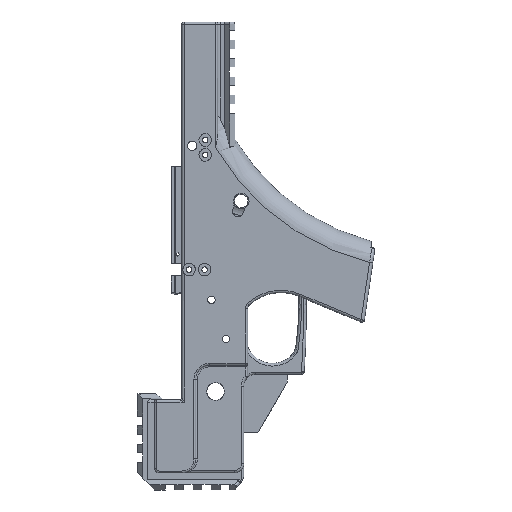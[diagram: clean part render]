
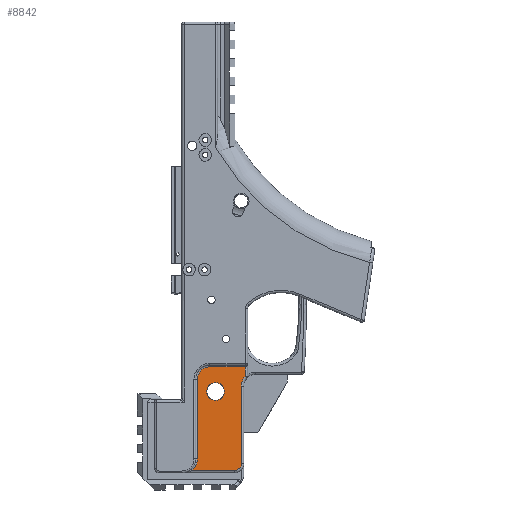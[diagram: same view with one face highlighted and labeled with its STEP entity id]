
A CAD part, left-side view. The second image highlights one B-rep face of the part: STEP entity #8842.
In plain terms, the highlighted planar face has unit normal (-1, 0, 0).
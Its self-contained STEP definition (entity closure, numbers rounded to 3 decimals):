
#143=FACE_BOUND('',#1619,.T.);
#611=CIRCLE('',#9327,7.62);
#613=CIRCLE('',#9331,3.81);
#632=CIRCLE('',#9359,6.752);
#637=CIRCLE('',#9367,8.488);
#704=CIRCLE('',#9526,4.826);
#1105=FACE_OUTER_BOUND('',#1618,.T.);
#1618=EDGE_LOOP('',(#6726,#6727,#6728,#6729,#6730,#6731,#6732,#6733,#6734));
#1619=EDGE_LOOP('',(#6735));
#2211=LINE('',#13867,#2984);
#2214=LINE('',#13884,#2987);
#2218=LINE('',#13924,#2991);
#2220=LINE('',#13937,#2993);
#2417=LINE('',#15144,#3190);
#2984=VECTOR('',#10611,10.);
#2987=VECTOR('',#10626,10.);
#2991=VECTOR('',#10670,10.);
#2993=VECTOR('',#10686,10.);
#3190=VECTOR('',#11211,10.);
#3818=VERTEX_POINT('',#13858);
#3820=VERTEX_POINT('',#13862);
#3821=VERTEX_POINT('',#13866);
#3823=VERTEX_POINT('',#13872);
#3825=VERTEX_POINT('',#13878);
#3840=VERTEX_POINT('',#13921);
#3841=VERTEX_POINT('',#13923);
#3843=VERTEX_POINT('',#13929);
#3845=VERTEX_POINT('',#13935);
#4061=VERTEX_POINT('',#15145);
#4747=EDGE_CURVE('',#3820,#3818,#611,.T.);
#4748=EDGE_CURVE('',#3818,#3821,#2211,.T.);
#4751=EDGE_CURVE('',#3821,#3823,#613,.T.);
#4756=EDGE_CURVE('',#3823,#3825,#2214,.T.);
#4773=EDGE_CURVE('',#3840,#3841,#2218,.T.);
#4777=EDGE_CURVE('',#3843,#3840,#632,.T.);
#4780=EDGE_CURVE('',#3845,#3843,#2220,.T.);
#4786=EDGE_CURVE('',#3825,#3845,#637,.T.);
#5090=EDGE_CURVE('',#3841,#3820,#2417,.T.);
#5091=EDGE_CURVE('',#4061,#4061,#704,.T.);
#6726=ORIENTED_EDGE('',*,*,#4747,.F.);
#6727=ORIENTED_EDGE('',*,*,#5090,.F.);
#6728=ORIENTED_EDGE('',*,*,#4773,.F.);
#6729=ORIENTED_EDGE('',*,*,#4777,.F.);
#6730=ORIENTED_EDGE('',*,*,#4780,.F.);
#6731=ORIENTED_EDGE('',*,*,#4786,.F.);
#6732=ORIENTED_EDGE('',*,*,#4756,.F.);
#6733=ORIENTED_EDGE('',*,*,#4751,.F.);
#6734=ORIENTED_EDGE('',*,*,#4748,.F.);
#6735=ORIENTED_EDGE('',*,*,#5091,.T.);
#8541=PLANE('',#9525);
#8842=ADVANCED_FACE('',(#1105,#143),#8541,.F.);
#9327=AXIS2_PLACEMENT_3D('',#13864,#10607,#10608);
#9331=AXIS2_PLACEMENT_3D('',#13873,#10617,#10618);
#9359=AXIS2_PLACEMENT_3D('',#13931,#10679,#10680);
#9367=AXIS2_PLACEMENT_3D('',#13970,#10698,#10699);
#9525=AXIS2_PLACEMENT_3D('',#15143,#11209,#11210);
#9526=AXIS2_PLACEMENT_3D('',#15146,#11212,#11213);
#10607=DIRECTION('center_axis',(-1.,0.,0.));
#10608=DIRECTION('ref_axis',(0.,0.928,0.373));
#10611=DIRECTION('',(0.,0.,-1.));
#10617=DIRECTION('center_axis',(1.,0.,0.));
#10618=DIRECTION('ref_axis',(0.,-0.707,-0.707));
#10626=DIRECTION('',(0.,1.,0.));
#10670=DIRECTION('',(0.,-1.,0.));
#10679=DIRECTION('center_axis',(1.,0.,0.));
#10680=DIRECTION('ref_axis',(0.,1.,0.));
#10686=DIRECTION('',(0.,0.,1.));
#10698=DIRECTION('center_axis',(-1.,0.,0.));
#10699=DIRECTION('ref_axis',(0.,-0.664,-0.748));
#11209=DIRECTION('center_axis',(1.,0.,0.));
#11210=DIRECTION('ref_axis',(0.,0.,-1.));
#11211=DIRECTION('',(0.,0.,-1.));
#11212=DIRECTION('center_axis',(1.,0.,0.));
#11213=DIRECTION('ref_axis',(0.,0.,-1.));
#13858=CARTESIAN_POINT('',(-11.43,-26.9,-130.907));
#13862=CARTESIAN_POINT('',(-11.43,-29.017,-125.636));
#13864=CARTESIAN_POINT('Origin',(-11.43,-34.52,-130.907));
#13866=CARTESIAN_POINT('',(-11.43,-26.9,-173.176));
#13867=CARTESIAN_POINT('',(-11.43,-26.9,-148.565));
#13872=CARTESIAN_POINT('',(-11.43,-23.09,-176.986));
#13873=CARTESIAN_POINT('Origin',(-11.43,-23.09,-173.176));
#13878=CARTESIAN_POINT('',(-11.43,-0.019,-176.986));
#13884=CARTESIAN_POINT('',(-11.43,-7.511,-176.986));
#13921=CARTESIAN_POINT('',(-11.43,-9.627,-120.454));
#13923=CARTESIAN_POINT('',(-11.43,-29.017,-120.454));
#13924=CARTESIAN_POINT('',(-11.43,-35.059,-120.454));
#13929=CARTESIAN_POINT('',(-11.43,-2.874,-127.206));
#13931=CARTESIAN_POINT('Origin',(-11.43,-9.627,-127.206));
#13935=CARTESIAN_POINT('',(-11.43,-2.874,-170.636));
#13937=CARTESIAN_POINT('',(-11.43,-2.874,-87.49));
#13970=CARTESIAN_POINT('Origin',(-11.43,5.613,-170.636));
#15143=CARTESIAN_POINT('Origin',(-11.43,-16.801,-129.514));
#15144=CARTESIAN_POINT('',(-11.43,-29.017,-161.99));
#15145=CARTESIAN_POINT('',(-11.43,-12.829,-129.103));
#15146=CARTESIAN_POINT('Origin',(-11.43,-12.829,-133.929));
